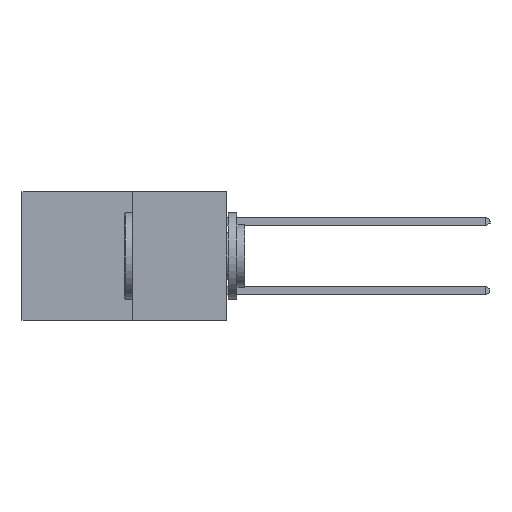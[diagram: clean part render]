
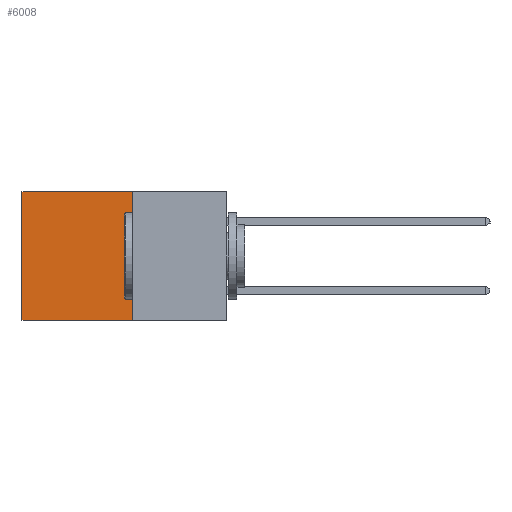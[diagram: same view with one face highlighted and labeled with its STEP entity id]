
A CAD part, left-side view. The second image highlights one B-rep face of the part: STEP entity #6008.
In plain terms, the highlighted planar face has unit normal (-1, 0, 0).
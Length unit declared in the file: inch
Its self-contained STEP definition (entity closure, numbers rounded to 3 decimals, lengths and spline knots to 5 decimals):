
#75 = EDGE_CURVE ( 'NONE', #666, #6654, #2656, .T. ) ;
#666 = VERTEX_POINT ( 'NONE', #4534 ) ;
#1163 = ORIENTED_EDGE ( 'NONE', *, *, #5142, .T. ) ;
#1673 = ORIENTED_EDGE ( 'NONE', *, *, #6479, .F. ) ;
#1984 = DIRECTION ( 'NONE',  ( 0., 0., -1. ) ) ;
#1999 = DIRECTION ( 'NONE',  ( 1., 0., 0. ) ) ;
#2009 = CARTESIAN_POINT ( 'NONE',  ( 0.277, 0.27, -0.37 ) ) ;
#2035 = PLANE ( 'NONE',  #3223 ) ;
#2317 = VERTEX_POINT ( 'NONE', #6319 ) ;
#2656 = LINE ( 'NONE', #3111, #2876 ) ;
#2707 = VECTOR ( 'NONE', #4717, 39.37008 ) ;
#2712 = EDGE_CURVE ( 'NONE', #3137, #2317, #8811, .T. ) ;
#2876 = VECTOR ( 'NONE', #3336, 39.37008 ) ;
#2924 = LINE ( 'NONE', #4795, #2707 ) ;
#3111 = CARTESIAN_POINT ( 'NONE',  ( 0.277, 0.27, -0.37 ) ) ;
#3137 = VERTEX_POINT ( 'NONE', #3376 ) ;
#3223 = AXIS2_PLACEMENT_3D ( 'NONE', #2009, #1999, #1984 ) ;
#3336 = DIRECTION ( 'NONE',  ( 0., 1., 0. ) ) ;
#3376 = CARTESIAN_POINT ( 'NONE',  ( 0.277, 0.27, 0. ) ) ;
#3379 = LINE ( 'NONE', #4462, #8989 ) ;
#3694 = ORIENTED_EDGE ( 'NONE', *, *, #2712, .T. ) ;
#4462 = CARTESIAN_POINT ( 'NONE',  ( 0.277, 0.27, -0.37 ) ) ;
#4534 = CARTESIAN_POINT ( 'NONE',  ( 0.277, 0.27, -0.37 ) ) ;
#4717 = DIRECTION ( 'NONE',  ( 0., 0., -1. ) ) ;
#4795 = CARTESIAN_POINT ( 'NONE',  ( 0.277, 0.59, -0.37 ) ) ;
#5142 = EDGE_CURVE ( 'NONE', #2317, #6654, #2924, .T. ) ;
#5172 = ORIENTED_EDGE ( 'NONE', *, *, #75, .F. ) ;
#5372 = CARTESIAN_POINT ( 'NONE',  ( 0.277, 0.59, -0.37 ) ) ;
#5420 = EDGE_LOOP ( 'NONE', ( #1163, #5172, #1673, #3694 ) ) ;
#6008 = ADVANCED_FACE ( 'NONE', ( #7141 ), #2035, .F. ) ;
#6319 = CARTESIAN_POINT ( 'NONE',  ( 0.277, 0.59, 0. ) ) ;
#6479 = EDGE_CURVE ( 'NONE', #3137, #666, #3379, .T. ) ;
#6654 = VERTEX_POINT ( 'NONE', #5372 ) ;
#6950 = VECTOR ( 'NONE', #7448, 39.37008 ) ;
#7141 = FACE_OUTER_BOUND ( 'NONE', #5420, .T. ) ;
#7371 = CARTESIAN_POINT ( 'NONE',  ( 0.277, 0.27, 0. ) ) ;
#7448 = DIRECTION ( 'NONE',  ( 0., 1., 0. ) ) ;
#8164 = DIRECTION ( 'NONE',  ( 0., 0., -1. ) ) ;
#8811 = LINE ( 'NONE', #7371, #6950 ) ;
#8989 = VECTOR ( 'NONE', #8164, 39.37008 ) ;
